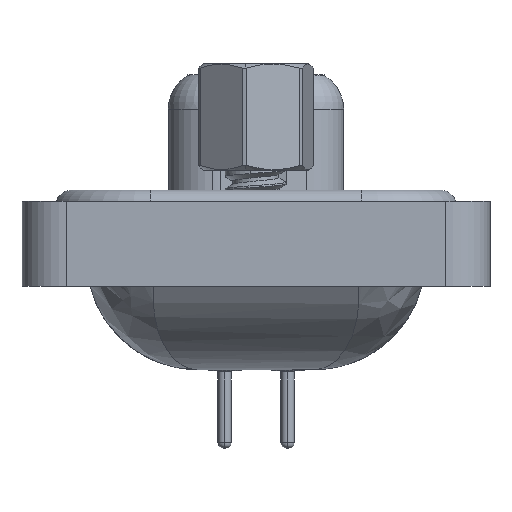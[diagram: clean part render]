
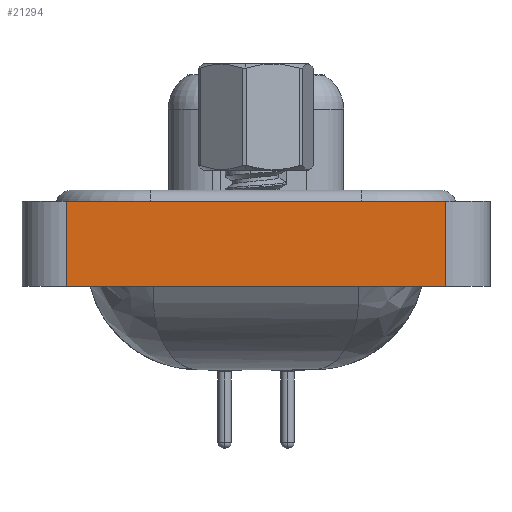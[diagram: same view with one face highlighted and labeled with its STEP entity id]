
A CAD part, left-side view. The second image highlights one B-rep face of the part: STEP entity #21294.
In plain terms, the highlighted planar face has unit normal (-1, 0, 0).
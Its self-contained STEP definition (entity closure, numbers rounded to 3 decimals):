
#397 = EDGE_CURVE ( 'NONE', #18075, #17812, #9595, .T. ) ;
#475 = DIRECTION ( 'NONE',  ( 0., -1., 0. ) ) ;
#1200 = ORIENTED_EDGE ( 'NONE', *, *, #13331, .T. ) ;
#2567 = DIRECTION ( 'NONE',  ( 0., 0., 1. ) ) ;
#3703 = ORIENTED_EDGE ( 'NONE', *, *, #5757, .F. ) ;
#4622 = EDGE_CURVE ( 'NONE', #18075, #17097, #7209, .T. ) ;
#4655 = VECTOR ( 'NONE', #18078, 1000. ) ;
#4804 = ORIENTED_EDGE ( 'NONE', *, *, #4622, .T. ) ;
#5143 = EDGE_LOOP ( 'NONE', ( #1200, #3703, #14050, #4804 ) ) ;
#5236 = VERTEX_POINT ( 'NONE', #13521 ) ;
#5757 = EDGE_CURVE ( 'NONE', #17812, #5236, #8664, .T. ) ;
#6526 = VECTOR ( 'NONE', #13571, 1000. ) ;
#7209 = LINE ( 'NONE', #13876, #8041 ) ;
#8041 = VECTOR ( 'NONE', #20516, 1000. ) ;
#8664 = LINE ( 'NONE', #15558, #15690 ) ;
#9327 = CARTESIAN_POINT ( 'NONE',  ( -7.25, -8.55, -3.35 ) ) ;
#9548 = CARTESIAN_POINT ( 'NONE',  ( -7.25, 8.55, 0.5 ) ) ;
#9595 = LINE ( 'NONE', #19719, #4655 ) ;
#10404 = LINE ( 'NONE', #11617, #6526 ) ;
#11617 = CARTESIAN_POINT ( 'NONE',  ( -7.25, -8.55, -3.35 ) ) ;
#12924 = FACE_OUTER_BOUND ( 'NONE', #5143, .T. ) ;
#13331 = EDGE_CURVE ( 'NONE', #17097, #5236, #10404, .T. ) ;
#13521 = CARTESIAN_POINT ( 'NONE',  ( -7.25, -8.55, 0.5 ) ) ;
#13571 = DIRECTION ( 'NONE',  ( 0., 0., 1. ) ) ;
#13876 = CARTESIAN_POINT ( 'NONE',  ( -7.25, -8.55, -3.35 ) ) ;
#14050 = ORIENTED_EDGE ( 'NONE', *, *, #397, .F. ) ;
#14678 = DIRECTION ( 'NONE',  ( -1., 0., 0. ) ) ;
#15558 = CARTESIAN_POINT ( 'NONE',  ( -7.25, -8.55, 0.5 ) ) ;
#15690 = VECTOR ( 'NONE', #475, 1000. ) ;
#17097 = VERTEX_POINT ( 'NONE', #21049 ) ;
#17812 = VERTEX_POINT ( 'NONE', #9548 ) ;
#17929 = CARTESIAN_POINT ( 'NONE',  ( -7.25, 8.55, -3.35 ) ) ;
#17992 = AXIS2_PLACEMENT_3D ( 'NONE', #9327, #14678, #2567 ) ;
#18075 = VERTEX_POINT ( 'NONE', #17929 ) ;
#18078 = DIRECTION ( 'NONE',  ( 0., 0., 1. ) ) ;
#19470 = PLANE ( 'NONE',  #17992 ) ;
#19719 = CARTESIAN_POINT ( 'NONE',  ( -7.25, 8.55, -3.35 ) ) ;
#20516 = DIRECTION ( 'NONE',  ( 0., -1., 0. ) ) ;
#21049 = CARTESIAN_POINT ( 'NONE',  ( -7.25, -8.55, -3.35 ) ) ;
#21294 = ADVANCED_FACE ( 'NONE', ( #12924 ), #19470, .T. ) ;
